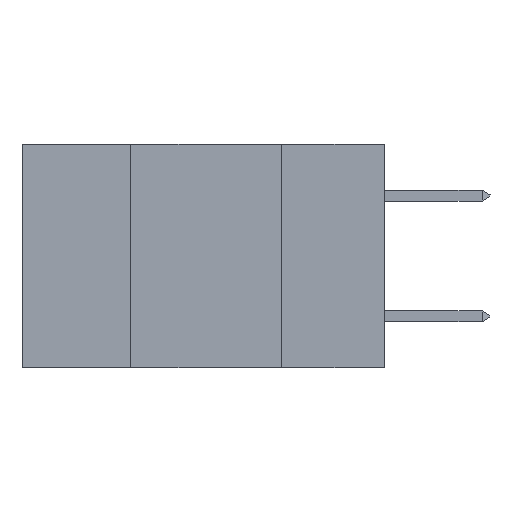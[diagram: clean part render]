
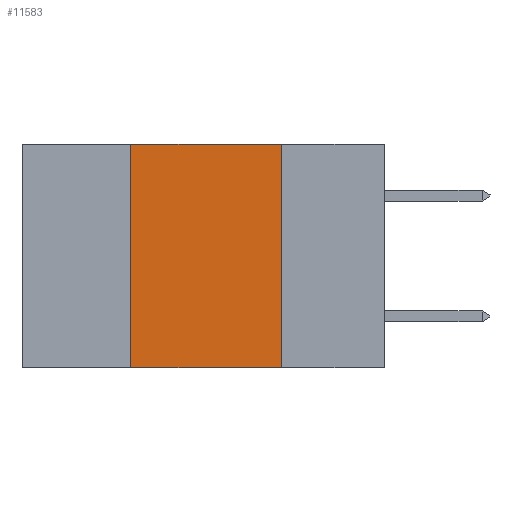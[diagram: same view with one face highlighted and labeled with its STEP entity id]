
A CAD part, left-side view. The second image highlights one B-rep face of the part: STEP entity #11583.
In plain terms, the highlighted planar face has unit normal (-1, 0, 0).
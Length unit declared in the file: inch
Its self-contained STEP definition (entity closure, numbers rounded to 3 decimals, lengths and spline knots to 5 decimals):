
#1909 = CARTESIAN_POINT ( 'NONE',  ( 0., 0.42, 0. ) ) ;
#4615 = ORIENTED_EDGE ( 'NONE', *, *, #11879, .F. ) ;
#4810 = DIRECTION ( 'NONE',  ( 0., -1., 0. ) ) ;
#5017 = AXIS2_PLACEMENT_3D ( 'NONE', #6170, #9305, #24550 ) ;
#5091 = EDGE_CURVE ( 'NONE', #10146, #9958, #24926, .T. ) ;
#6170 = CARTESIAN_POINT ( 'NONE',  ( 0., 0.6, 0. ) ) ;
#8546 = LINE ( 'NONE', #34676, #19845 ) ;
#8942 = VECTOR ( 'NONE', #19042, 39.37008 ) ;
#9305 = DIRECTION ( 'NONE',  ( 1., 0., 0. ) ) ;
#9958 = VERTEX_POINT ( 'NONE', #22921 ) ;
#10146 = VERTEX_POINT ( 'NONE', #23313 ) ;
#11583 = ADVANCED_FACE ( 'NONE', ( #29722 ), #30588, .F. ) ;
#11879 = EDGE_CURVE ( 'NONE', #33714, #10146, #8546, .T. ) ;
#12835 = LINE ( 'NONE', #26218, #19867 ) ;
#15564 = EDGE_CURVE ( 'NONE', #21681, #33714, #28959, .T. ) ;
#19042 = DIRECTION ( 'NONE',  ( 0., 0., -1. ) ) ;
#19845 = VECTOR ( 'NONE', #4810, 39.37008 ) ;
#19867 = VECTOR ( 'NONE', #32281, 39.37008 ) ;
#20933 = EDGE_CURVE ( 'NONE', #21681, #9958, #12835, .T. ) ;
#21681 = VERTEX_POINT ( 'NONE', #32514 ) ;
#22921 = CARTESIAN_POINT ( 'NONE',  ( 0., 0.17, -0.37 ) ) ;
#23313 = CARTESIAN_POINT ( 'NONE',  ( 0., 0.17, 0. ) ) ;
#23978 = ORIENTED_EDGE ( 'NONE', *, *, #5091, .F. ) ;
#24251 = VECTOR ( 'NONE', #37684, 39.37008 ) ;
#24550 = DIRECTION ( 'NONE',  ( 0., 0., -1. ) ) ;
#24711 = CARTESIAN_POINT ( 'NONE',  ( 0., 0.17, 0. ) ) ;
#24926 = LINE ( 'NONE', #24711, #8942 ) ;
#26218 = CARTESIAN_POINT ( 'NONE',  ( 0., 0.6, -0.37 ) ) ;
#28194 = CARTESIAN_POINT ( 'NONE',  ( 0., 0.42, 0. ) ) ;
#28959 = LINE ( 'NONE', #1909, #24251 ) ;
#29722 = FACE_OUTER_BOUND ( 'NONE', #35731, .T. ) ;
#30588 = PLANE ( 'NONE',  #5017 ) ;
#31210 = ORIENTED_EDGE ( 'NONE', *, *, #15564, .F. ) ;
#32281 = DIRECTION ( 'NONE',  ( 0., -1., 0. ) ) ;
#32514 = CARTESIAN_POINT ( 'NONE',  ( 0., 0.42, -0.37 ) ) ;
#33714 = VERTEX_POINT ( 'NONE', #28194 ) ;
#34615 = ORIENTED_EDGE ( 'NONE', *, *, #20933, .T. ) ;
#34676 = CARTESIAN_POINT ( 'NONE',  ( 0., 0.6, 0. ) ) ;
#35731 = EDGE_LOOP ( 'NONE', ( #23978, #4615, #31210, #34615 ) ) ;
#37684 = DIRECTION ( 'NONE',  ( 0., 0., 1. ) ) ;
